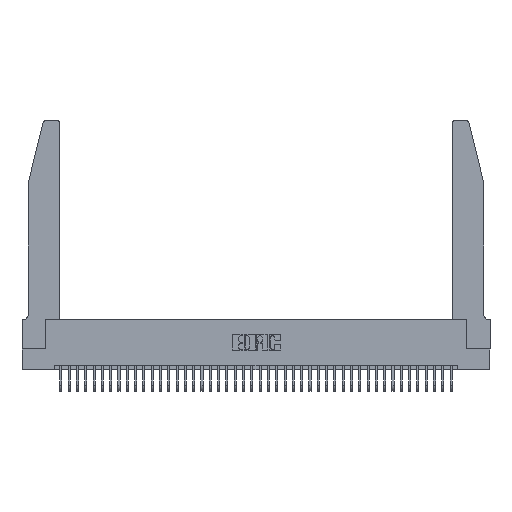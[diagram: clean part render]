
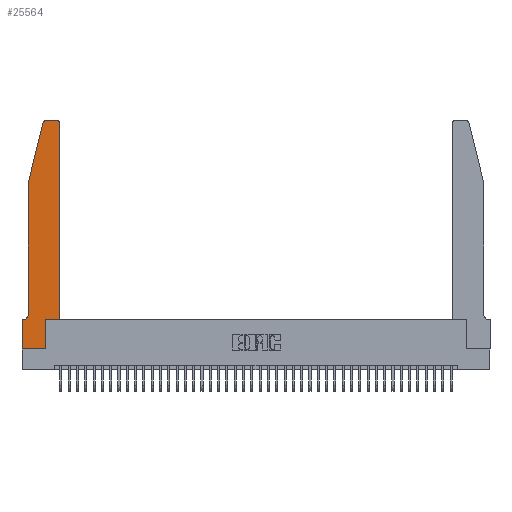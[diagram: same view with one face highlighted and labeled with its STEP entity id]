
A CAD part, top view. The second image highlights one B-rep face of the part: STEP entity #25564.
In plain terms, the highlighted planar face has unit normal (0, 0, 1).
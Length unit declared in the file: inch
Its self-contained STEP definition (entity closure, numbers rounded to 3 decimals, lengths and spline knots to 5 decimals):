
#42 = CARTESIAN_POINT ( 'NONE',  ( 0., 0.35, 0.37 ) ) ;
#139 = VECTOR ( 'NONE', #13483, 39.37008 ) ;
#814 = ORIENTED_EDGE ( 'NONE', *, *, #13143, .T. ) ;
#1641 = CARTESIAN_POINT ( 'NONE',  ( 0.4505, 0.35, 0.37 ) ) ;
#1834 = ORIENTED_EDGE ( 'NONE', *, *, #38010, .T. ) ;
#1931 = DIRECTION ( 'NONE',  ( -0.239, -0.971, 0. ) ) ;
#2657 = CARTESIAN_POINT ( 'NONE',  ( 0.4505, 2.72, 0.37 ) ) ;
#2750 = CARTESIAN_POINT ( 'NONE',  ( 0.4505, 0.35, 0.37 ) ) ;
#2953 = ORIENTED_EDGE ( 'NONE', *, *, #30846, .T. ) ;
#3001 = ORIENTED_EDGE ( 'NONE', *, *, #8188, .T. ) ;
#3179 = DIRECTION ( 'NONE',  ( 0., 1., 0. ) ) ;
#3920 = CARTESIAN_POINT ( 'NONE',  ( 0.4205, 2.75, 0.37 ) ) ;
#3949 = EDGE_CURVE ( 'NONE', #34400, #4940, #22272, .T. ) ;
#3986 = VECTOR ( 'NONE', #6823, 39.37008 ) ;
#4049 = DIRECTION ( 'NONE',  ( 0., 0., 1. ) ) ;
#4568 = VERTEX_POINT ( 'NONE', #3920 ) ;
#4940 = VERTEX_POINT ( 'NONE', #2657 ) ;
#4955 = CARTESIAN_POINT ( 'NONE',  ( 0.2865, 0.35, 0.37 ) ) ;
#5478 = AXIS2_PLACEMENT_3D ( 'NONE', #22596, #4049, #25716 ) ;
#6267 = VERTEX_POINT ( 'NONE', #33272 ) ;
#6597 = VERTEX_POINT ( 'NONE', #38395 ) ;
#6823 = DIRECTION ( 'NONE',  ( -1., 0., 0. ) ) ;
#6974 = VECTOR ( 'NONE', #33082, 39.37008 ) ;
#7051 = CARTESIAN_POINT ( 'NONE',  ( 0., 0., 0.37 ) ) ;
#7101 = CARTESIAN_POINT ( 'NONE',  ( 0.4505, 0.35, 0.37 ) ) ;
#8166 = VERTEX_POINT ( 'NONE', #25359 ) ;
#8188 = EDGE_CURVE ( 'NONE', #4568, #6597, #22391, .T. ) ;
#8445 = VERTEX_POINT ( 'NONE', #11163 ) ;
#8855 = EDGE_CURVE ( 'NONE', #4940, #4568, #29661, .T. ) ;
#8959 = ORIENTED_EDGE ( 'NONE', *, *, #8855, .T. ) ;
#10392 = CARTESIAN_POINT ( 'NONE',  ( 0.0755, 2., 0.37 ) ) ;
#10908 = LINE ( 'NONE', #29686, #34547 ) ;
#11087 = ORIENTED_EDGE ( 'NONE', *, *, #25651, .T. ) ;
#11163 = CARTESIAN_POINT ( 'NONE',  ( 0.2865, 0.35, 0.37 ) ) ;
#11867 = VECTOR ( 'NONE', #33472, 39.37008 ) ;
#13143 = EDGE_CURVE ( 'NONE', #37566, #18253, #38996, .T. ) ;
#13483 = DIRECTION ( 'NONE',  ( 0., -1., 0. ) ) ;
#13673 = DIRECTION ( 'NONE',  ( 0., -1., 0. ) ) ;
#14019 = CARTESIAN_POINT ( 'NONE',  ( 0.0055, 0.42, 0.37 ) ) ;
#14042 = VERTEX_POINT ( 'NONE', #42 ) ;
#14064 = VECTOR ( 'NONE', #3179, 39.37008 ) ;
#14449 = VECTOR ( 'NONE', #22513, 39.37008 ) ;
#14462 = EDGE_CURVE ( 'NONE', #8166, #30284, #31643, .T. ) ;
#14754 = AXIS2_PLACEMENT_3D ( 'NONE', #19161, #16159, #37794 ) ;
#16159 = DIRECTION ( 'NONE',  ( 0., 0., 1. ) ) ;
#17101 = DIRECTION ( 'NONE',  ( -1., 0., 0. ) ) ;
#18253 = VERTEX_POINT ( 'NONE', #37898 ) ;
#18549 = DIRECTION ( 'NONE',  ( 0., 0., 1. ) ) ;
#19161 = CARTESIAN_POINT ( 'NONE',  ( 0., 0.35, 0.37 ) ) ;
#20636 = DIRECTION ( 'NONE',  ( 0., 1., 0. ) ) ;
#20671 = CARTESIAN_POINT ( 'NONE',  ( 0., 0., 0.37 ) ) ;
#20717 = ORIENTED_EDGE ( 'NONE', *, *, #25845, .T. ) ;
#21158 = ORIENTED_EDGE ( 'NONE', *, *, #3949, .T. ) ;
#21376 = EDGE_CURVE ( 'NONE', #6597, #6267, #39950, .T. ) ;
#22272 = LINE ( 'NONE', #2750, #14064 ) ;
#22391 = LINE ( 'NONE', #28456, #3986 ) ;
#22513 = DIRECTION ( 'NONE',  ( 1., 0., 0. ) ) ;
#22596 = CARTESIAN_POINT ( 'NONE',  ( 0.4205, 2.72, 0.37 ) ) ;
#23866 = VERTEX_POINT ( 'NONE', #37543 ) ;
#24310 = CARTESIAN_POINT ( 'NONE',  ( 0.0755, 0.35, 0.37 ) ) ;
#25247 = EDGE_LOOP ( 'NONE', ( #3001, #34894, #31496, #11087, #814, #2953, #1834, #37164, #20717, #33338, #21158, #8959 ) ) ;
#25359 = CARTESIAN_POINT ( 'NONE',  ( 0., 0., 0.37 ) ) ;
#25393 = VECTOR ( 'NONE', #20636, 39.37008 ) ;
#25564 = ADVANCED_FACE ( 'NONE', ( #27820 ), #31584, .T. ) ;
#25651 = EDGE_CURVE ( 'NONE', #23866, #37566, #33123, .T. ) ;
#25716 = DIRECTION ( 'NONE',  ( 1., 0., 0. ) ) ;
#25835 = EDGE_CURVE ( 'NONE', #6267, #23866, #10908, .T. ) ;
#25845 = EDGE_CURVE ( 'NONE', #30284, #8445, #26359, .T. ) ;
#26359 = LINE ( 'NONE', #4955, #25393 ) ;
#27820 = FACE_OUTER_BOUND ( 'NONE', #25247, .T. ) ;
#28456 = CARTESIAN_POINT ( 'NONE',  ( 0.2605, 2.75, 0.37 ) ) ;
#29271 = LINE ( 'NONE', #24310, #11867 ) ;
#29383 = VECTOR ( 'NONE', #13673, 39.37008 ) ;
#29661 = CIRCLE ( 'NONE', #5478, 0.03 ) ;
#29686 = CARTESIAN_POINT ( 'NONE',  ( 0.0755, 2., 0.37 ) ) ;
#30284 = VERTEX_POINT ( 'NONE', #40134 ) ;
#30340 = LINE ( 'NONE', #7051, #29383 ) ;
#30846 = EDGE_CURVE ( 'NONE', #18253, #14042, #29271, .T. ) ;
#31393 = AXIS2_PLACEMENT_3D ( 'NONE', #37060, #18549, #40165 ) ;
#31496 = ORIENTED_EDGE ( 'NONE', *, *, #25835, .T. ) ;
#31584 = PLANE ( 'NONE',  #14754 ) ;
#31643 = LINE ( 'NONE', #20671, #6974 ) ;
#33024 = CARTESIAN_POINT ( 'NONE',  ( 0.0755, 0.42, 0.37 ) ) ;
#33082 = DIRECTION ( 'NONE',  ( 1., 0., 0. ) ) ;
#33123 = LINE ( 'NONE', #10392, #139 ) ;
#33272 = CARTESIAN_POINT ( 'NONE',  ( 0.25487, 2.72718, 0.37 ) ) ;
#33338 = ORIENTED_EDGE ( 'NONE', *, *, #37293, .T. ) ;
#33472 = DIRECTION ( 'NONE',  ( -1., 0., 0. ) ) ;
#34400 = VERTEX_POINT ( 'NONE', #1641 ) ;
#34547 = VECTOR ( 'NONE', #1931, 39.37008 ) ;
#34894 = ORIENTED_EDGE ( 'NONE', *, *, #21376, .T. ) ;
#35625 = DIRECTION ( 'NONE',  ( 0., 0., -1. ) ) ;
#37060 = CARTESIAN_POINT ( 'NONE',  ( 0.284, 2.72, 0.37 ) ) ;
#37164 = ORIENTED_EDGE ( 'NONE', *, *, #14462, .T. ) ;
#37293 = EDGE_CURVE ( 'NONE', #8445, #34400, #39095, .T. ) ;
#37543 = CARTESIAN_POINT ( 'NONE',  ( 0.0755, 2., 0.37 ) ) ;
#37566 = VERTEX_POINT ( 'NONE', #33024 ) ;
#37644 = AXIS2_PLACEMENT_3D ( 'NONE', #14019, #35625, #17101 ) ;
#37794 = DIRECTION ( 'NONE',  ( 1., 0., 0. ) ) ;
#37898 = CARTESIAN_POINT ( 'NONE',  ( 0.0055, 0.35, 0.37 ) ) ;
#38010 = EDGE_CURVE ( 'NONE', #14042, #8166, #30340, .T. ) ;
#38395 = CARTESIAN_POINT ( 'NONE',  ( 0.284, 2.75, 0.37 ) ) ;
#38996 = CIRCLE ( 'NONE', #37644, 0.07 ) ;
#39095 = LINE ( 'NONE', #7101, #14449 ) ;
#39950 = CIRCLE ( 'NONE', #31393, 0.03 ) ;
#40134 = CARTESIAN_POINT ( 'NONE',  ( 0.2865, 0., 0.37 ) ) ;
#40165 = DIRECTION ( 'NONE',  ( 1., 0., 0. ) ) ;
